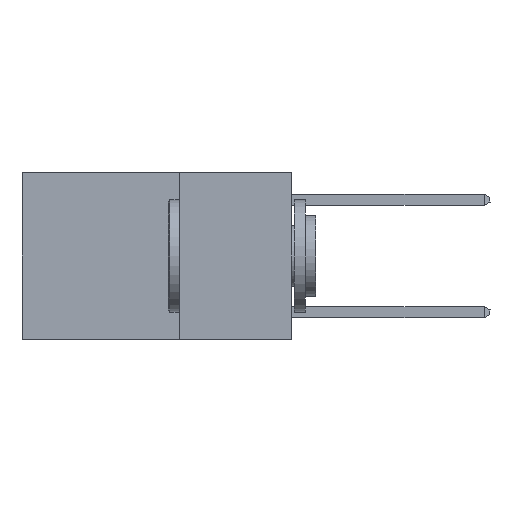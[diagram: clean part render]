
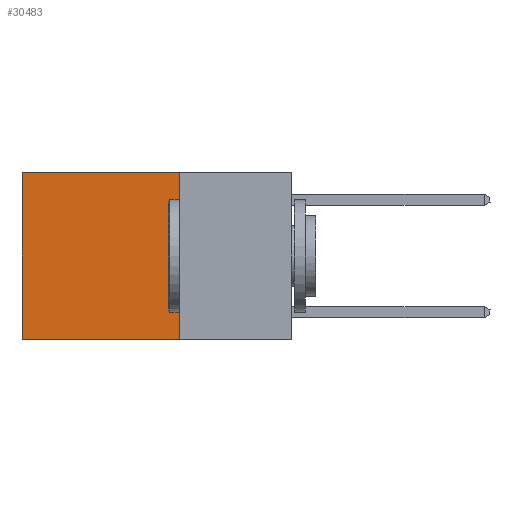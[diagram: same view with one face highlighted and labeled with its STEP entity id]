
A CAD part, left-side view. The second image highlights one B-rep face of the part: STEP entity #30483.
In plain terms, the highlighted planar face has unit normal (-1, 0, 0).
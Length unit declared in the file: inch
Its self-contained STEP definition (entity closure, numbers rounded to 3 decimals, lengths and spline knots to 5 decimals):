
#584 = CARTESIAN_POINT ( 'NONE',  ( 0.2625, 0.6, 0. ) ) ;
#1175 = CARTESIAN_POINT ( 'NONE',  ( 0.2625, 0.25, -0.37 ) ) ;
#1830 = EDGE_CURVE ( 'NONE', #17156, #11976, #7431, .T. ) ;
#4127 = EDGE_CURVE ( 'NONE', #28256, #20869, #11987, .T. ) ;
#4947 = EDGE_CURVE ( 'NONE', #20869, #11976, #18122, .T. ) ;
#5148 = EDGE_LOOP ( 'NONE', ( #28609, #17470, #22728, #5573 ) ) ;
#5310 = CARTESIAN_POINT ( 'NONE',  ( 0.2625, 0.25, 0. ) ) ;
#5382 = CARTESIAN_POINT ( 'NONE',  ( 0.2625, 0.25, -0.37 ) ) ;
#5573 = ORIENTED_EDGE ( 'NONE', *, *, #12918, .T. ) ;
#6922 = VECTOR ( 'NONE', #16629, 39.37008 ) ;
#7340 = DIRECTION ( 'NONE',  ( 1., 0., 0. ) ) ;
#7431 = LINE ( 'NONE', #7591, #19702 ) ;
#7591 = CARTESIAN_POINT ( 'NONE',  ( 0.2625, 0.6, 0. ) ) ;
#9152 = LINE ( 'NONE', #18742, #28300 ) ;
#11976 = VERTEX_POINT ( 'NONE', #21850 ) ;
#11987 = LINE ( 'NONE', #14468, #6922 ) ;
#12918 = EDGE_CURVE ( 'NONE', #28256, #17156, #9152, .T. ) ;
#14468 = CARTESIAN_POINT ( 'NONE',  ( 0.2625, 0.25, 0. ) ) ;
#14609 = PLANE ( 'NONE',  #19194 ) ;
#14767 = FACE_OUTER_BOUND ( 'NONE', #5148, .T. ) ;
#16629 = DIRECTION ( 'NONE',  ( 0., 0., -1. ) ) ;
#17156 = VERTEX_POINT ( 'NONE', #584 ) ;
#17470 = ORIENTED_EDGE ( 'NONE', *, *, #4947, .F. ) ;
#18122 = LINE ( 'NONE', #1175, #18298 ) ;
#18298 = VECTOR ( 'NONE', #25390, 39.37008 ) ;
#18742 = CARTESIAN_POINT ( 'NONE',  ( 0.2625, 0.25, 0. ) ) ;
#19194 = AXIS2_PLACEMENT_3D ( 'NONE', #5310, #7340, #24223 ) ;
#19702 = VECTOR ( 'NONE', #28488, 39.37008 ) ;
#20869 = VERTEX_POINT ( 'NONE', #5382 ) ;
#21850 = CARTESIAN_POINT ( 'NONE',  ( 0.2625, 0.6, -0.37 ) ) ;
#22728 = ORIENTED_EDGE ( 'NONE', *, *, #4127, .F. ) ;
#23551 = CARTESIAN_POINT ( 'NONE',  ( 0.2625, 0.25, 0. ) ) ;
#24223 = DIRECTION ( 'NONE',  ( 0., 0., -1. ) ) ;
#25390 = DIRECTION ( 'NONE',  ( 0., 1., 0. ) ) ;
#28195 = DIRECTION ( 'NONE',  ( 0., 1., 0. ) ) ;
#28256 = VERTEX_POINT ( 'NONE', #23551 ) ;
#28300 = VECTOR ( 'NONE', #28195, 39.37008 ) ;
#28488 = DIRECTION ( 'NONE',  ( 0., 0., -1. ) ) ;
#28609 = ORIENTED_EDGE ( 'NONE', *, *, #1830, .T. ) ;
#30483 = ADVANCED_FACE ( 'NONE', ( #14767 ), #14609, .F. ) ;
